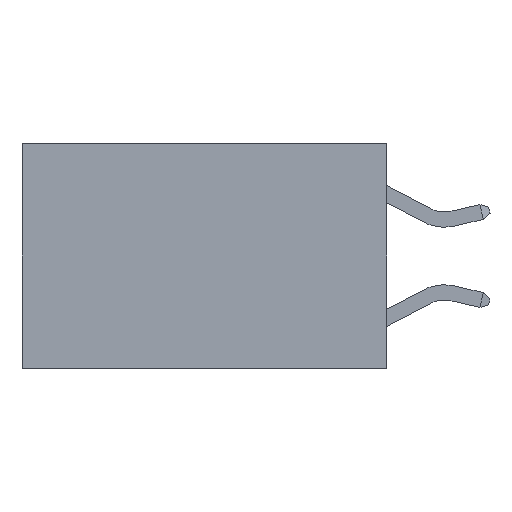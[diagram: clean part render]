
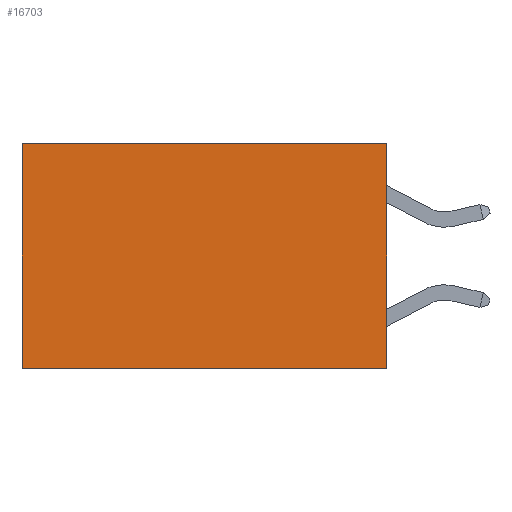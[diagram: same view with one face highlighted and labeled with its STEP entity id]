
A CAD part, left-side view. The second image highlights one B-rep face of the part: STEP entity #16703.
In plain terms, the highlighted planar face has unit normal (-1, 0, 0).
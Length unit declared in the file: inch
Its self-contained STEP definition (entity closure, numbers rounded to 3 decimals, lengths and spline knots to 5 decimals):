
#1456 = DIRECTION ( 'NONE',  ( 0., 0., -1. ) ) ;
#1517 = CARTESIAN_POINT ( 'NONE',  ( 0.2625, 0., 0. ) ) ;
#1905 = CARTESIAN_POINT ( 'NONE',  ( 0.2625, 0.6, 0. ) ) ;
#2168 = CARTESIAN_POINT ( 'NONE',  ( 0.2625, 0.6, 0. ) ) ;
#2414 = ORIENTED_EDGE ( 'NONE', *, *, #3951, .T. ) ;
#3047 = CARTESIAN_POINT ( 'NONE',  ( 0.2625, 0., -0.37 ) ) ;
#3129 = VECTOR ( 'NONE', #10500, 39.37008 ) ;
#3558 = EDGE_CURVE ( 'NONE', #13312, #7166, #13066, .T. ) ;
#3951 = EDGE_CURVE ( 'NONE', #8431, #13312, #14325, .T. ) ;
#4416 = DIRECTION ( 'NONE',  ( 0., 1., 0. ) ) ;
#4419 = LINE ( 'NONE', #1517, #11192 ) ;
#4780 = DIRECTION ( 'NONE',  ( 0., 0., -1. ) ) ;
#5198 = PLANE ( 'NONE',  #15485 ) ;
#5890 = VECTOR ( 'NONE', #4780, 39.37008 ) ;
#6396 = CARTESIAN_POINT ( 'NONE',  ( 0.2625, 0., -0.37 ) ) ;
#6518 = CARTESIAN_POINT ( 'NONE',  ( 0.2625, 0., 0. ) ) ;
#7166 = VERTEX_POINT ( 'NONE', #14973 ) ;
#7879 = DIRECTION ( 'NONE',  ( 1., 0., 0. ) ) ;
#8431 = VERTEX_POINT ( 'NONE', #8802 ) ;
#8758 = ORIENTED_EDGE ( 'NONE', *, *, #3558, .T. ) ;
#8802 = CARTESIAN_POINT ( 'NONE',  ( 0.2625, 0., 0. ) ) ;
#9350 = VERTEX_POINT ( 'NONE', #6396 ) ;
#9592 = EDGE_CURVE ( 'NONE', #8431, #9350, #4419, .T. ) ;
#9646 = EDGE_CURVE ( 'NONE', #9350, #7166, #13921, .T. ) ;
#9752 = CARTESIAN_POINT ( 'NONE',  ( 0.2625, 0., 0. ) ) ;
#9933 = FACE_OUTER_BOUND ( 'NONE', #10845, .T. ) ;
#10500 = DIRECTION ( 'NONE',  ( 0., 1., 0. ) ) ;
#10845 = EDGE_LOOP ( 'NONE', ( #8758, #12389, #13816, #2414 ) ) ;
#11192 = VECTOR ( 'NONE', #1456, 39.37008 ) ;
#12389 = ORIENTED_EDGE ( 'NONE', *, *, #9646, .F. ) ;
#13066 = LINE ( 'NONE', #1905, #5890 ) ;
#13312 = VERTEX_POINT ( 'NONE', #2168 ) ;
#13816 = ORIENTED_EDGE ( 'NONE', *, *, #9592, .F. ) ;
#13921 = LINE ( 'NONE', #3047, #14333 ) ;
#14325 = LINE ( 'NONE', #9752, #3129 ) ;
#14333 = VECTOR ( 'NONE', #4416, 39.37008 ) ;
#14973 = CARTESIAN_POINT ( 'NONE',  ( 0.2625, 0.6, -0.37 ) ) ;
#15485 = AXIS2_PLACEMENT_3D ( 'NONE', #6518, #7879, #17325 ) ;
#16703 = ADVANCED_FACE ( 'NONE', ( #9933 ), #5198, .F. ) ;
#17325 = DIRECTION ( 'NONE',  ( 0., 0., -1. ) ) ;
